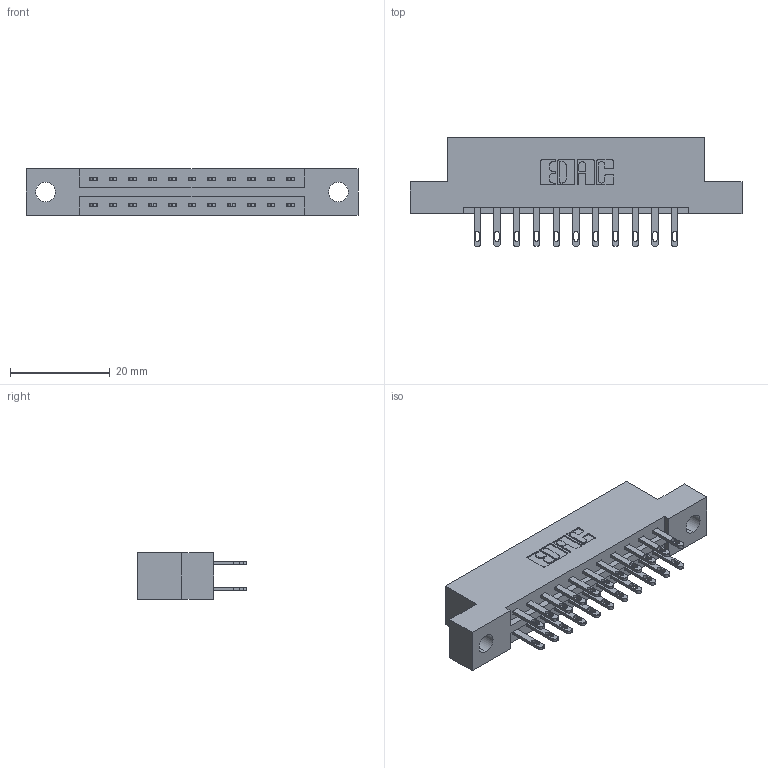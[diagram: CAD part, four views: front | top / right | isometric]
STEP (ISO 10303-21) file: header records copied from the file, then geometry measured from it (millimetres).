
FILE_DESCRIPTION (( 'STEP AP203' ), '1' );
FILE_NAME ('887-022-500-204.STEP', '2020-09-20T18:36:22', ( '' ), ( '' ), 'SwSTEP 2.0', 'SolidWorks 2020', '' );
FILE_SCHEMA (( 'CONFIG_CONTROL_DESIGN' ));
Length unit declared in the file: inch
Products named in the file (3): 887-022-500-204; 345-292-001_345-293-100; 837 Part_Flush Mounting Lugs - 0.156 Dia-TH
Assembly tree (23 placements, depth 2):
  887-022-500-204
    837 Part_Flush Mounting Lugs - 0.156 Dia-TH
    345-292-001_345-293-100  x22
Bounding box: 66.6 x 21.85 x 9.4 mm (x, y, z)
Volume: 6585.4 mm3; surface area: 7185.2 mm2
Topology: 23 solids, 23 shells, 1214 faces, 3677 edges, 2450 vertices
Faces by surface type: plane 774, cylinder 440
Entity records: 12471 total; most frequent: CARTESIAN_POINT 2126, ORIENTED_EDGE 2062, DIRECTION 1867, EDGE_CURVE 1031, LINE 899, VECTOR 899, VERTEX_POINT 686, AXIS2_PLACEMENT_3D 484
